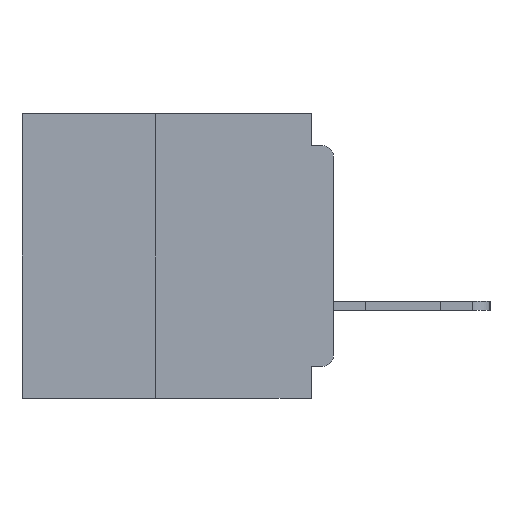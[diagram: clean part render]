
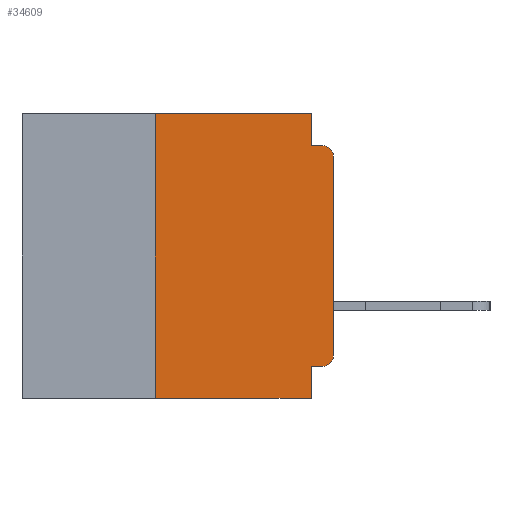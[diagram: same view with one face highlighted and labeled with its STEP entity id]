
A CAD part, left-side view. The second image highlights one B-rep face of the part: STEP entity #34609.
In plain terms, the highlighted planar face has unit normal (-1, 0, 0).
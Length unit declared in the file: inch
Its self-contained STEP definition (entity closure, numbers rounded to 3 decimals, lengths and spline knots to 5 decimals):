
#1655 = EDGE_CURVE ( 'NONE', #12941, #2013, #11484, .T. ) ;
#1707 = VECTOR ( 'NONE', #39782, 39.37008 ) ;
#1912 = LINE ( 'NONE', #43081, #11131 ) ;
#2013 = VERTEX_POINT ( 'NONE', #28757 ) ;
#2745 = FACE_OUTER_BOUND ( 'NONE', #19203, .T. ) ;
#3567 = AXIS2_PLACEMENT_3D ( 'NONE', #28853, #8271, #32281 ) ;
#3685 = LINE ( 'NONE', #22185, #30054 ) ;
#3851 = ORIENTED_EDGE ( 'NONE', *, *, #37869, .T. ) ;
#4181 = VERTEX_POINT ( 'NONE', #18194 ) ;
#4576 = VERTEX_POINT ( 'NONE', #8920 ) ;
#5455 = VERTEX_POINT ( 'NONE', #24871 ) ;
#6587 = CARTESIAN_POINT ( 'NONE',  ( 0., 0.031, -0.355 ) ) ;
#7591 = LINE ( 'NONE', #19238, #15701 ) ;
#7994 = PLANE ( 'NONE',  #41996 ) ;
#8069 = CARTESIAN_POINT ( 'NONE',  ( 0., 0., -0.34 ) ) ;
#8271 = DIRECTION ( 'NONE',  ( -1., 0., 0. ) ) ;
#8284 = ORIENTED_EDGE ( 'NONE', *, *, #38276, .F. ) ;
#8606 = LINE ( 'NONE', #14877, #25877 ) ;
#8811 = DIRECTION ( 'NONE',  ( 0., -1., 0. ) ) ;
#8920 = CARTESIAN_POINT ( 'NONE',  ( 0., 0.031, 0. ) ) ;
#9281 = EDGE_CURVE ( 'NONE', #4576, #31580, #3685, .T. ) ;
#10632 = ORIENTED_EDGE ( 'NONE', *, *, #9281, .F. ) ;
#11131 = VECTOR ( 'NONE', #22591, 39.37008 ) ;
#11231 = VERTEX_POINT ( 'NONE', #14763 ) ;
#11319 = CARTESIAN_POINT ( 'NONE',  ( 0., 0.437, 0. ) ) ;
#11477 = DIRECTION ( 'NONE',  ( 0., 0., -1. ) ) ;
#11484 = CIRCLE ( 'NONE', #20871, 0.015 ) ;
#12172 = VERTEX_POINT ( 'NONE', #36986 ) ;
#12941 = VERTEX_POINT ( 'NONE', #34066 ) ;
#14762 = CARTESIAN_POINT ( 'NONE',  ( 0., 0.031, -0.045 ) ) ;
#14763 = CARTESIAN_POINT ( 'NONE',  ( 0., 0.25, -0.4 ) ) ;
#14877 = CARTESIAN_POINT ( 'NONE',  ( 0., 0., -0.045 ) ) ;
#15701 = VECTOR ( 'NONE', #8811, 39.37008 ) ;
#15999 = LINE ( 'NONE', #23038, #42284 ) ;
#17195 = CARTESIAN_POINT ( 'NONE',  ( 0., 0., -0.355 ) ) ;
#18194 = CARTESIAN_POINT ( 'NONE',  ( 0., 0.031, -0.4 ) ) ;
#18354 = DIRECTION ( 'NONE',  ( 0., -1., 0. ) ) ;
#19203 = EDGE_LOOP ( 'NONE', ( #37632, #26221, #8284, #10632, #23962, #44401, #3851, #34322, #40958, #39864 ) ) ;
#19238 = CARTESIAN_POINT ( 'NONE',  ( 0., 0.437, 0. ) ) ;
#20088 = LINE ( 'NONE', #36286, #1707 ) ;
#20871 = AXIS2_PLACEMENT_3D ( 'NONE', #35434, #36096, #36149 ) ;
#22185 = CARTESIAN_POINT ( 'NONE',  ( 0., 0.031, 0. ) ) ;
#22278 = VECTOR ( 'NONE', #44505, 39.37008 ) ;
#22532 = VERTEX_POINT ( 'NONE', #6587 ) ;
#22591 = DIRECTION ( 'NONE',  ( 0., 0., 1. ) ) ;
#22952 = CIRCLE ( 'NONE', #3567, 0.015 ) ;
#23038 = CARTESIAN_POINT ( 'NONE',  ( 0., 0.031, -0.4 ) ) ;
#23962 = ORIENTED_EDGE ( 'NONE', *, *, #27457, .F. ) ;
#24871 = CARTESIAN_POINT ( 'NONE',  ( 0., 0.015, -0.355 ) ) ;
#25617 = DIRECTION ( 'NONE',  ( 0., 0., -1. ) ) ;
#25877 = VECTOR ( 'NONE', #18354, 39.37008 ) ;
#26221 = ORIENTED_EDGE ( 'NONE', *, *, #1655, .T. ) ;
#27457 = EDGE_CURVE ( 'NONE', #12172, #4576, #7591, .T. ) ;
#28757 = CARTESIAN_POINT ( 'NONE',  ( 0., 0.015, -0.045 ) ) ;
#28853 = CARTESIAN_POINT ( 'NONE',  ( 0., 0.015, -0.34 ) ) ;
#30054 = VECTOR ( 'NONE', #25617, 39.37008 ) ;
#30379 = VERTEX_POINT ( 'NONE', #8069 ) ;
#31580 = VERTEX_POINT ( 'NONE', #14762 ) ;
#31990 = DIRECTION ( 'NONE',  ( 1., 0., 0. ) ) ;
#32281 = DIRECTION ( 'NONE',  ( 0., 0., -1. ) ) ;
#33559 = EDGE_CURVE ( 'NONE', #30379, #12941, #20088, .T. ) ;
#33876 = VECTOR ( 'NONE', #40119, 39.37008 ) ;
#34066 = CARTESIAN_POINT ( 'NONE',  ( 0., 0., -0.06 ) ) ;
#34322 = ORIENTED_EDGE ( 'NONE', *, *, #40266, .F. ) ;
#34609 = ADVANCED_FACE ( 'NONE', ( #2745 ), #7994, .F. ) ;
#34956 = LINE ( 'NONE', #36624, #33876 ) ;
#35434 = CARTESIAN_POINT ( 'NONE',  ( 0., 0.015, -0.06 ) ) ;
#36096 = DIRECTION ( 'NONE',  ( -1., 0., 0. ) ) ;
#36149 = DIRECTION ( 'NONE',  ( 0., 0., -1. ) ) ;
#36286 = CARTESIAN_POINT ( 'NONE',  ( 0., 0., 0. ) ) ;
#36432 = DIRECTION ( 'NONE',  ( 0., 0., -1. ) ) ;
#36624 = CARTESIAN_POINT ( 'NONE',  ( 0., 0.437, -0.4 ) ) ;
#36872 = EDGE_CURVE ( 'NONE', #5455, #22532, #40459, .T. ) ;
#36986 = CARTESIAN_POINT ( 'NONE',  ( 0., 0.25, 0. ) ) ;
#37632 = ORIENTED_EDGE ( 'NONE', *, *, #33559, .T. ) ;
#37869 = EDGE_CURVE ( 'NONE', #11231, #4181, #34956, .T. ) ;
#38276 = EDGE_CURVE ( 'NONE', #31580, #2013, #8606, .T. ) ;
#39782 = DIRECTION ( 'NONE',  ( 0., 0., 1. ) ) ;
#39864 = ORIENTED_EDGE ( 'NONE', *, *, #41847, .T. ) ;
#40119 = DIRECTION ( 'NONE',  ( 0., -1., 0. ) ) ;
#40148 = EDGE_CURVE ( 'NONE', #11231, #12172, #1912, .T. ) ;
#40266 = EDGE_CURVE ( 'NONE', #22532, #4181, #15999, .T. ) ;
#40459 = LINE ( 'NONE', #17195, #22278 ) ;
#40958 = ORIENTED_EDGE ( 'NONE', *, *, #36872, .F. ) ;
#41847 = EDGE_CURVE ( 'NONE', #5455, #30379, #22952, .T. ) ;
#41996 = AXIS2_PLACEMENT_3D ( 'NONE', #11319, #31990, #11477 ) ;
#42284 = VECTOR ( 'NONE', #36432, 39.37008 ) ;
#43081 = CARTESIAN_POINT ( 'NONE',  ( 0., 0.25, -0.4 ) ) ;
#44401 = ORIENTED_EDGE ( 'NONE', *, *, #40148, .F. ) ;
#44505 = DIRECTION ( 'NONE',  ( 0., 1., 0. ) ) ;
